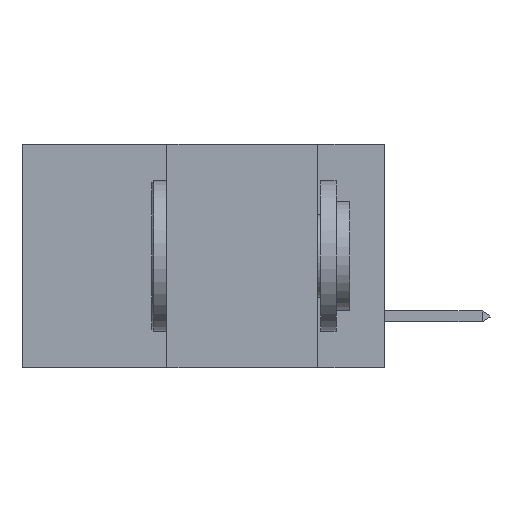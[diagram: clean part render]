
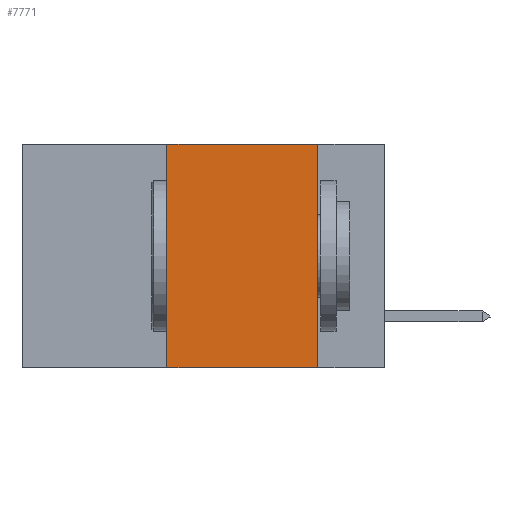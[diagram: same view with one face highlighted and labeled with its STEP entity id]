
A CAD part, left-side view. The second image highlights one B-rep face of the part: STEP entity #7771.
In plain terms, the highlighted planar face has unit normal (-1, 0, 0).
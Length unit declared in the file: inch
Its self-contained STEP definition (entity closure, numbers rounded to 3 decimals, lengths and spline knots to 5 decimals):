
#516 = VECTOR ( 'NONE', #3017, 39.37008 ) ;
#1106 = CARTESIAN_POINT ( 'NONE',  ( 0., 0.36, 0. ) ) ;
#2093 = FACE_OUTER_BOUND ( 'NONE', #8955, .T. ) ;
#2757 = EDGE_CURVE ( 'NONE', #10216, #5798, #14841, .T. ) ;
#2922 = VECTOR ( 'NONE', #7396, 39.37008 ) ;
#3017 = DIRECTION ( 'NONE',  ( 0., -1., 0. ) ) ;
#3574 = CARTESIAN_POINT ( 'NONE',  ( 0., 0.11, -0.37 ) ) ;
#4742 = VECTOR ( 'NONE', #8614, 39.37008 ) ;
#4829 = VERTEX_POINT ( 'NONE', #3574 ) ;
#5152 = VERTEX_POINT ( 'NONE', #12923 ) ;
#5798 = VERTEX_POINT ( 'NONE', #1106 ) ;
#5816 = CARTESIAN_POINT ( 'NONE',  ( 0., 0.6, 0. ) ) ;
#6032 = LINE ( 'NONE', #8682, #2922 ) ;
#6267 = LINE ( 'NONE', #12447, #7529 ) ;
#6704 = ORIENTED_EDGE ( 'NONE', *, *, #9577, .F. ) ;
#7014 = DIRECTION ( 'NONE',  ( 0., 0., -1. ) ) ;
#7396 = DIRECTION ( 'NONE',  ( 0., -1., 0. ) ) ;
#7529 = VECTOR ( 'NONE', #11158, 39.37008 ) ;
#7771 = ADVANCED_FACE ( 'NONE', ( #2093 ), #10771, .F. ) ;
#8614 = DIRECTION ( 'NONE',  ( 0., 0., 1. ) ) ;
#8682 = CARTESIAN_POINT ( 'NONE',  ( 0., 0.6, -0.37 ) ) ;
#8820 = ORIENTED_EDGE ( 'NONE', *, *, #10935, .F. ) ;
#8955 = EDGE_LOOP ( 'NONE', ( #6704, #8820, #14757, #10794 ) ) ;
#9571 = DIRECTION ( 'NONE',  ( 1., 0., 0. ) ) ;
#9577 = EDGE_CURVE ( 'NONE', #5152, #4829, #6267, .T. ) ;
#9896 = LINE ( 'NONE', #12271, #516 ) ;
#10216 = VERTEX_POINT ( 'NONE', #15077 ) ;
#10491 = EDGE_CURVE ( 'NONE', #10216, #4829, #6032, .T. ) ;
#10696 = AXIS2_PLACEMENT_3D ( 'NONE', #5816, #9571, #7014 ) ;
#10771 = PLANE ( 'NONE',  #10696 ) ;
#10794 = ORIENTED_EDGE ( 'NONE', *, *, #10491, .T. ) ;
#10935 = EDGE_CURVE ( 'NONE', #5798, #5152, #9896, .T. ) ;
#11144 = CARTESIAN_POINT ( 'NONE',  ( 0., 0.36, 0. ) ) ;
#11158 = DIRECTION ( 'NONE',  ( 0., 0., -1. ) ) ;
#12271 = CARTESIAN_POINT ( 'NONE',  ( 0., 0.6, 0. ) ) ;
#12447 = CARTESIAN_POINT ( 'NONE',  ( 0., 0.11, 0. ) ) ;
#12923 = CARTESIAN_POINT ( 'NONE',  ( 0., 0.11, 0. ) ) ;
#14757 = ORIENTED_EDGE ( 'NONE', *, *, #2757, .F. ) ;
#14841 = LINE ( 'NONE', #11144, #4742 ) ;
#15077 = CARTESIAN_POINT ( 'NONE',  ( 0., 0.36, -0.37 ) ) ;
